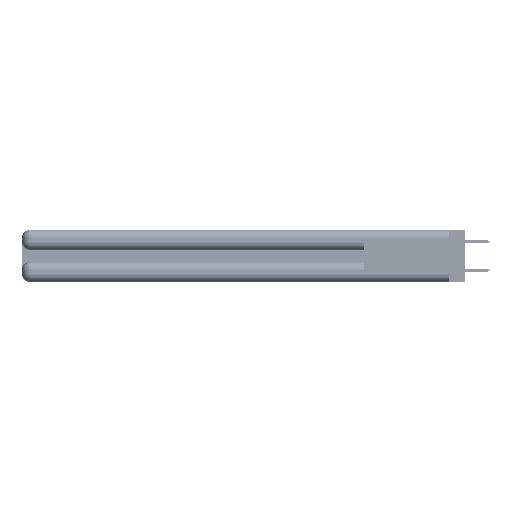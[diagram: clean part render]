
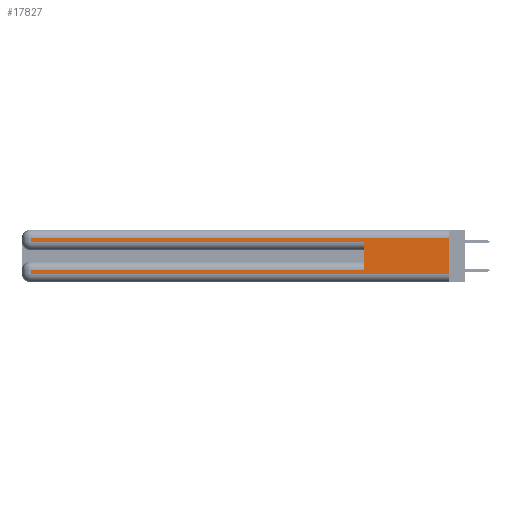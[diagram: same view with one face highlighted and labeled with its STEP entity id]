
A CAD part, left-side view. The second image highlights one B-rep face of the part: STEP entity #17827.
In plain terms, the highlighted planar face has unit normal (-1, 0, 0).
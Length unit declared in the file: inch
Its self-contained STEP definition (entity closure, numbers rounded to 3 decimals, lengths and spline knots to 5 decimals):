
#645 = CARTESIAN_POINT ( 'NONE',  ( 0., 2.94, 0.085 ) ) ;
#855 = ORIENTED_EDGE ( 'NONE', *, *, #45554, .T. ) ;
#1340 = LINE ( 'NONE', #6245, #3870 ) ;
#1891 = DIRECTION ( 'NONE',  ( 0., 1., 0. ) ) ;
#3504 = AXIS2_PLACEMENT_3D ( 'NONE', #42721, #46959, #22905 ) ;
#3870 = VECTOR ( 'NONE', #30371, 39.37008 ) ;
#4118 = DIRECTION ( 'NONE',  ( 0., -1., 0. ) ) ;
#5639 = ORIENTED_EDGE ( 'NONE', *, *, #28858, .T. ) ;
#6245 = CARTESIAN_POINT ( 'NONE',  ( 0., 0., 0.37 ) ) ;
#7044 = VERTEX_POINT ( 'NONE', #19181 ) ;
#7347 = CARTESIAN_POINT ( 'NONE',  ( 0., 0.6, 0.085 ) ) ;
#8083 = VECTOR ( 'NONE', #33307, 39.37008 ) ;
#8533 = ORIENTED_EDGE ( 'NONE', *, *, #9757, .F. ) ;
#9368 = CARTESIAN_POINT ( 'NONE',  ( 0., 0.6, 0.145 ) ) ;
#9757 = EDGE_CURVE ( 'NONE', #11801, #34670, #1340, .T. ) ;
#9825 = CARTESIAN_POINT ( 'NONE',  ( 0., 0., 0.31 ) ) ;
#10061 = ORIENTED_EDGE ( 'NONE', *, *, #38139, .T. ) ;
#11211 = EDGE_CURVE ( 'NONE', #35813, #38128, #42669, .T. ) ;
#11801 = VERTEX_POINT ( 'NONE', #33619 ) ;
#14157 = LINE ( 'NONE', #48038, #23617 ) ;
#16287 = VECTOR ( 'NONE', #17197, 39.37008 ) ;
#17197 = DIRECTION ( 'NONE',  ( 0., 0., -1. ) ) ;
#17476 = LINE ( 'NONE', #46002, #23136 ) ;
#17827 = ADVANCED_FACE ( 'NONE', ( #34064 ), #42897, .F. ) ;
#18242 = VERTEX_POINT ( 'NONE', #645 ) ;
#19181 = CARTESIAN_POINT ( 'NONE',  ( 0., 2.94, 0.06 ) ) ;
#21452 = VECTOR ( 'NONE', #41975, 39.37008 ) ;
#22905 = DIRECTION ( 'NONE',  ( 0., 0., -1. ) ) ;
#23136 = VECTOR ( 'NONE', #1891, 39.37008 ) ;
#23272 = EDGE_CURVE ( 'NONE', #47269, #38128, #51137, .T. ) ;
#23617 = VECTOR ( 'NONE', #52044, 39.37008 ) ;
#25136 = CARTESIAN_POINT ( 'NONE',  ( 0., 2.94, 0.37 ) ) ;
#26303 = EDGE_LOOP ( 'NONE', ( #8533, #855, #32329, #39078, #28997, #10061, #5639, #33494 ) ) ;
#28858 = EDGE_CURVE ( 'NONE', #18242, #7044, #48386, .T. ) ;
#28997 = ORIENTED_EDGE ( 'NONE', *, *, #11211, .F. ) ;
#30371 = DIRECTION ( 'NONE',  ( 0., 0., -1. ) ) ;
#31726 = CARTESIAN_POINT ( 'NONE',  ( 0., 2.94, 0.31 ) ) ;
#32130 = LINE ( 'NONE', #9825, #21452 ) ;
#32329 = ORIENTED_EDGE ( 'NONE', *, *, #48752, .T. ) ;
#33307 = DIRECTION ( 'NONE',  ( 0., 0., 1. ) ) ;
#33494 = ORIENTED_EDGE ( 'NONE', *, *, #47444, .T. ) ;
#33619 = CARTESIAN_POINT ( 'NONE',  ( 0., 0., 0.31 ) ) ;
#34064 = FACE_OUTER_BOUND ( 'NONE', #26303, .T. ) ;
#34670 = VERTEX_POINT ( 'NONE', #47217 ) ;
#35813 = VERTEX_POINT ( 'NONE', #7347 ) ;
#37931 = CARTESIAN_POINT ( 'NONE',  ( 0., 0.6, 0.285 ) ) ;
#38128 = VERTEX_POINT ( 'NONE', #37931 ) ;
#38139 = EDGE_CURVE ( 'NONE', #35813, #18242, #17476, .T. ) ;
#38475 = CARTESIAN_POINT ( 'NONE',  ( 0., 0., 0.06 ) ) ;
#39078 = ORIENTED_EDGE ( 'NONE', *, *, #23272, .T. ) ;
#40455 = VECTOR ( 'NONE', #4118, 39.37008 ) ;
#41293 = CARTESIAN_POINT ( 'NONE',  ( 0., 2.94, 0.285 ) ) ;
#41975 = DIRECTION ( 'NONE',  ( 0., 1., 0. ) ) ;
#42504 = DIRECTION ( 'NONE',  ( 0., -1., 0. ) ) ;
#42588 = VERTEX_POINT ( 'NONE', #31726 ) ;
#42669 = LINE ( 'NONE', #9368, #8083 ) ;
#42721 = CARTESIAN_POINT ( 'NONE',  ( 0., 0., 0.37 ) ) ;
#42897 = PLANE ( 'NONE',  #3504 ) ;
#45554 = EDGE_CURVE ( 'NONE', #11801, #42588, #32130, .T. ) ;
#46002 = CARTESIAN_POINT ( 'NONE',  ( 0., 0., 0.085 ) ) ;
#46959 = DIRECTION ( 'NONE',  ( 1., 0., 0. ) ) ;
#47217 = CARTESIAN_POINT ( 'NONE',  ( 0., 0., 0.06 ) ) ;
#47269 = VERTEX_POINT ( 'NONE', #41293 ) ;
#47444 = EDGE_CURVE ( 'NONE', #7044, #34670, #52004, .T. ) ;
#48038 = CARTESIAN_POINT ( 'NONE',  ( 0., 2.94, 0.37 ) ) ;
#48386 = LINE ( 'NONE', #25136, #16287 ) ;
#48752 = EDGE_CURVE ( 'NONE', #42588, #47269, #14157, .T. ) ;
#49472 = CARTESIAN_POINT ( 'NONE',  ( 0., 0., 0.285 ) ) ;
#50752 = VECTOR ( 'NONE', #42504, 39.37008 ) ;
#51137 = LINE ( 'NONE', #49472, #40455 ) ;
#52004 = LINE ( 'NONE', #38475, #50752 ) ;
#52044 = DIRECTION ( 'NONE',  ( 0., 0., -1. ) ) ;
